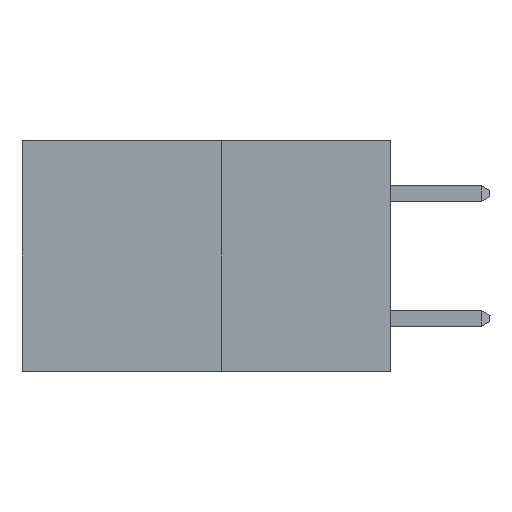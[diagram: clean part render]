
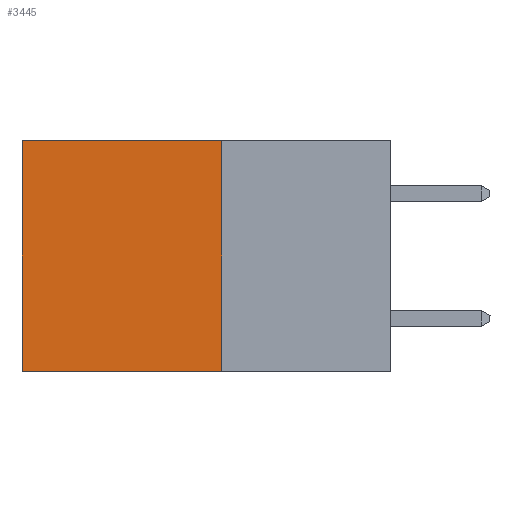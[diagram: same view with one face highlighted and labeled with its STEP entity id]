
A CAD part, left-side view. The second image highlights one B-rep face of the part: STEP entity #3445.
In plain terms, the highlighted planar face has unit normal (-1, 0, 0).
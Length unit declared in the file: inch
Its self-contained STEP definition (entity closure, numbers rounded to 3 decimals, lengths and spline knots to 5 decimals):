
#484 = EDGE_CURVE ( 'NONE', #8934, #1604, #5513, .T. ) ;
#601 = DIRECTION ( 'NONE',  ( 0., 0., -1. ) ) ;
#711 = AXIS2_PLACEMENT_3D ( 'NONE', #2913, #743, #3822 ) ;
#743 = DIRECTION ( 'NONE',  ( 1., 0., 0. ) ) ;
#744 = CARTESIAN_POINT ( 'NONE',  ( 0.277, 0.27, 0. ) ) ;
#979 = PLANE ( 'NONE',  #711 ) ;
#1006 = EDGE_CURVE ( 'NONE', #3355, #8934, #5138, .T. ) ;
#1498 = EDGE_LOOP ( 'NONE', ( #9425, #6371, #5013, #5194 ) ) ;
#1584 = CARTESIAN_POINT ( 'NONE',  ( 0.277, 0.59, 0. ) ) ;
#1604 = VERTEX_POINT ( 'NONE', #7188 ) ;
#1930 = FACE_OUTER_BOUND ( 'NONE', #1498, .T. ) ;
#2063 = CARTESIAN_POINT ( 'NONE',  ( 0.277, 0.27, -0.37 ) ) ;
#2102 = CARTESIAN_POINT ( 'NONE',  ( 0.277, 0.27, -0.37 ) ) ;
#2763 = VECTOR ( 'NONE', #7185, 39.37008 ) ;
#2768 = LINE ( 'NONE', #3829, #4895 ) ;
#2913 = CARTESIAN_POINT ( 'NONE',  ( 0.277, 0.27, -0.37 ) ) ;
#3088 = DIRECTION ( 'NONE',  ( 0., 1., 0. ) ) ;
#3355 = VERTEX_POINT ( 'NONE', #744 ) ;
#3445 = ADVANCED_FACE ( 'NONE', ( #1930 ), #979, .F. ) ;
#3822 = DIRECTION ( 'NONE',  ( 0., 0., -1. ) ) ;
#3829 = CARTESIAN_POINT ( 'NONE',  ( 0.277, 0.27, 0. ) ) ;
#4702 = DIRECTION ( 'NONE',  ( 0., 1., 0. ) ) ;
#4895 = VECTOR ( 'NONE', #4702, 39.37008 ) ;
#5013 = ORIENTED_EDGE ( 'NONE', *, *, #1006, .F. ) ;
#5138 = LINE ( 'NONE', #5708, #2763 ) ;
#5194 = ORIENTED_EDGE ( 'NONE', *, *, #6392, .T. ) ;
#5214 = CARTESIAN_POINT ( 'NONE',  ( 0.277, 0.59, -0.37 ) ) ;
#5281 = VECTOR ( 'NONE', #3088, 39.37008 ) ;
#5513 = LINE ( 'NONE', #2102, #5281 ) ;
#5708 = CARTESIAN_POINT ( 'NONE',  ( 0.277, 0.27, -0.37 ) ) ;
#6371 = ORIENTED_EDGE ( 'NONE', *, *, #484, .F. ) ;
#6392 = EDGE_CURVE ( 'NONE', #3355, #8324, #2768, .T. ) ;
#7185 = DIRECTION ( 'NONE',  ( 0., 0., -1. ) ) ;
#7188 = CARTESIAN_POINT ( 'NONE',  ( 0.277, 0.59, -0.37 ) ) ;
#7358 = VECTOR ( 'NONE', #601, 39.37008 ) ;
#8316 = EDGE_CURVE ( 'NONE', #8324, #1604, #9338, .T. ) ;
#8324 = VERTEX_POINT ( 'NONE', #1584 ) ;
#8934 = VERTEX_POINT ( 'NONE', #2063 ) ;
#9338 = LINE ( 'NONE', #5214, #7358 ) ;
#9425 = ORIENTED_EDGE ( 'NONE', *, *, #8316, .T. ) ;
